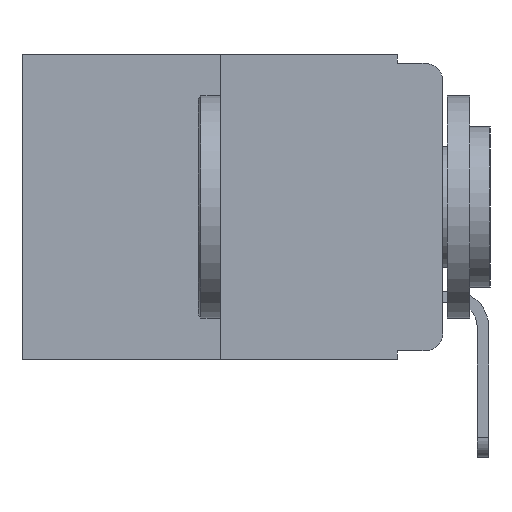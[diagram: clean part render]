
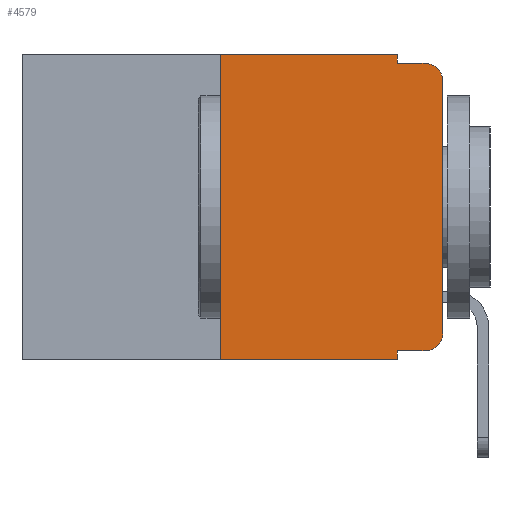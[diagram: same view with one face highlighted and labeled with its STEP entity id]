
A CAD part, left-side view. The second image highlights one B-rep face of the part: STEP entity #4579.
In plain terms, the highlighted planar face has unit normal (-1, 0, 0).
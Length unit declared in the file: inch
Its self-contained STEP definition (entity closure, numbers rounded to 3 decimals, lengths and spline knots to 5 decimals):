
#309 = LINE ( 'NONE', #5500, #14558 ) ;
#513 = LINE ( 'NONE', #11163, #12330 ) ;
#767 = CARTESIAN_POINT ( 'NONE',  ( 0., 0.02, -0.03 ) ) ;
#893 = EDGE_CURVE ( 'NONE', #6931, #13372, #2261, .T. ) ;
#1354 = ORIENTED_EDGE ( 'NONE', *, *, #10127, .F. ) ;
#1369 = EDGE_CURVE ( 'NONE', #12546, #5245, #14546, .T. ) ;
#1867 = AXIS2_PLACEMENT_3D ( 'NONE', #14423, #15904, #11700 ) ;
#1891 = VERTEX_POINT ( 'NONE', #10132 ) ;
#2036 = CARTESIAN_POINT ( 'NONE',  ( 0., 0.25, 0. ) ) ;
#2261 = LINE ( 'NONE', #15724, #11966 ) ;
#2540 = VERTEX_POINT ( 'NONE', #10116 ) ;
#2576 = ORIENTED_EDGE ( 'NONE', *, *, #4516, .F. ) ;
#2583 = EDGE_CURVE ( 'NONE', #13372, #12142, #3004, .T. ) ;
#2898 = ORIENTED_EDGE ( 'NONE', *, *, #8900, .F. ) ;
#3004 = CIRCLE ( 'NONE', #1867, 0.02 ) ;
#3499 = DIRECTION ( 'NONE',  ( 0., -1., 0. ) ) ;
#3804 = CARTESIAN_POINT ( 'NONE',  ( 0., 0.051, 0. ) ) ;
#4201 = CARTESIAN_POINT ( 'NONE',  ( 0., 0.051, -0.01 ) ) ;
#4516 = EDGE_CURVE ( 'NONE', #6931, #2540, #309, .T. ) ;
#4579 = ADVANCED_FACE ( 'NONE', ( #8477 ), #13857, .F. ) ;
#4760 = CARTESIAN_POINT ( 'NONE',  ( 0., 0., 0. ) ) ;
#5245 = VERTEX_POINT ( 'NONE', #4201 ) ;
#5500 = CARTESIAN_POINT ( 'NONE',  ( 0., 0.051, 0. ) ) ;
#5634 = EDGE_CURVE ( 'NONE', #8429, #11711, #10692, .T. ) ;
#5805 = DIRECTION ( 'NONE',  ( 0., 0., 1. ) ) ;
#6041 = DIRECTION ( 'NONE',  ( -1., 0., 0. ) ) ;
#6113 = AXIS2_PLACEMENT_3D ( 'NONE', #6722, #12110, #14825 ) ;
#6181 = EDGE_CURVE ( 'NONE', #8429, #2540, #12119, .T. ) ;
#6722 = CARTESIAN_POINT ( 'NONE',  ( 0., 0.473, 0. ) ) ;
#6931 = VERTEX_POINT ( 'NONE', #11642 ) ;
#7044 = AXIS2_PLACEMENT_3D ( 'NONE', #767, #6041, #11511 ) ;
#7326 = CARTESIAN_POINT ( 'NONE',  ( 0., 0., -0.03 ) ) ;
#8133 = VERTEX_POINT ( 'NONE', #7326 ) ;
#8394 = DIRECTION ( 'NONE',  ( 0., 0., -1. ) ) ;
#8429 = VERTEX_POINT ( 'NONE', #16555 ) ;
#8434 = EDGE_CURVE ( 'NONE', #12142, #8133, #9778, .T. ) ;
#8477 = FACE_OUTER_BOUND ( 'NONE', #16725, .T. ) ;
#8900 = EDGE_CURVE ( 'NONE', #11711, #12546, #513, .T. ) ;
#9357 = ORIENTED_EDGE ( 'NONE', *, *, #8434, .T. ) ;
#9778 = LINE ( 'NONE', #4760, #14003 ) ;
#9936 = CARTESIAN_POINT ( 'NONE',  ( 0., 0.051, -0.01 ) ) ;
#10116 = CARTESIAN_POINT ( 'NONE',  ( 0., 0.051, -0.343 ) ) ;
#10127 = EDGE_CURVE ( 'NONE', #5245, #1891, #13813, .T. ) ;
#10132 = CARTESIAN_POINT ( 'NONE',  ( 0., 0.02, -0.01 ) ) ;
#10223 = ORIENTED_EDGE ( 'NONE', *, *, #893, .T. ) ;
#10437 = DIRECTION ( 'NONE',  ( 0., 0., 1. ) ) ;
#10692 = LINE ( 'NONE', #16058, #15564 ) ;
#11163 = CARTESIAN_POINT ( 'NONE',  ( 0., 0.473, 0. ) ) ;
#11255 = DIRECTION ( 'NONE',  ( 0., -1., 0. ) ) ;
#11496 = ORIENTED_EDGE ( 'NONE', *, *, #5634, .F. ) ;
#11511 = DIRECTION ( 'NONE',  ( 0., 0., -1. ) ) ;
#11642 = CARTESIAN_POINT ( 'NONE',  ( 0., 0.051, -0.333 ) ) ;
#11700 = DIRECTION ( 'NONE',  ( 0., 0., -1. ) ) ;
#11711 = VERTEX_POINT ( 'NONE', #2036 ) ;
#11966 = VECTOR ( 'NONE', #3499, 39.37008 ) ;
#12102 = EDGE_CURVE ( 'NONE', #8133, #1891, #14634, .T. ) ;
#12110 = DIRECTION ( 'NONE',  ( 1., 0., 0. ) ) ;
#12119 = LINE ( 'NONE', #15103, #15499 ) ;
#12142 = VERTEX_POINT ( 'NONE', #13095 ) ;
#12330 = VECTOR ( 'NONE', #11255, 39.37008 ) ;
#12454 = ORIENTED_EDGE ( 'NONE', *, *, #2583, .T. ) ;
#12546 = VERTEX_POINT ( 'NONE', #16513 ) ;
#12973 = DIRECTION ( 'NONE',  ( 0., 0., -1. ) ) ;
#13095 = CARTESIAN_POINT ( 'NONE',  ( 0., 0., -0.313 ) ) ;
#13372 = VERTEX_POINT ( 'NONE', #14972 ) ;
#13521 = DIRECTION ( 'NONE',  ( 0., -1., 0. ) ) ;
#13813 = LINE ( 'NONE', #9936, #14052 ) ;
#13857 = PLANE ( 'NONE',  #6113 ) ;
#13878 = ORIENTED_EDGE ( 'NONE', *, *, #12102, .T. ) ;
#13897 = ORIENTED_EDGE ( 'NONE', *, *, #1369, .F. ) ;
#14003 = VECTOR ( 'NONE', #5805, 39.37008 ) ;
#14052 = VECTOR ( 'NONE', #15303, 39.37008 ) ;
#14211 = VECTOR ( 'NONE', #12973, 39.37008 ) ;
#14423 = CARTESIAN_POINT ( 'NONE',  ( 0., 0.02, -0.313 ) ) ;
#14546 = LINE ( 'NONE', #3804, #14211 ) ;
#14558 = VECTOR ( 'NONE', #8394, 39.37008 ) ;
#14634 = CIRCLE ( 'NONE', #7044, 0.02 ) ;
#14825 = DIRECTION ( 'NONE',  ( 0., 0., -1. ) ) ;
#14972 = CARTESIAN_POINT ( 'NONE',  ( 0., 0.02, -0.333 ) ) ;
#15103 = CARTESIAN_POINT ( 'NONE',  ( 0., 0.473, -0.343 ) ) ;
#15303 = DIRECTION ( 'NONE',  ( 0., -1., 0. ) ) ;
#15499 = VECTOR ( 'NONE', #13521, 39.37008 ) ;
#15564 = VECTOR ( 'NONE', #10437, 39.37008 ) ;
#15724 = CARTESIAN_POINT ( 'NONE',  ( 0., 0.051, -0.333 ) ) ;
#15904 = DIRECTION ( 'NONE',  ( -1., 0., 0. ) ) ;
#16058 = CARTESIAN_POINT ( 'NONE',  ( 0., 0.25, 0. ) ) ;
#16513 = CARTESIAN_POINT ( 'NONE',  ( 0., 0.051, 0. ) ) ;
#16555 = CARTESIAN_POINT ( 'NONE',  ( 0., 0.25, -0.343 ) ) ;
#16725 = EDGE_LOOP ( 'NONE', ( #9357, #13878, #1354, #13897, #2898, #11496, #17296, #2576, #10223, #12454 ) ) ;
#17296 = ORIENTED_EDGE ( 'NONE', *, *, #6181, .T. ) ;
